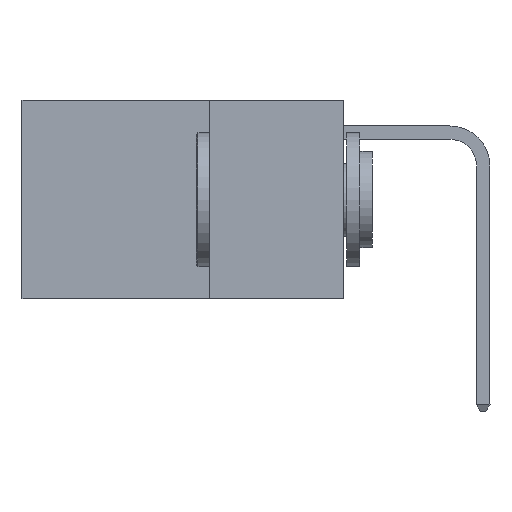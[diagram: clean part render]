
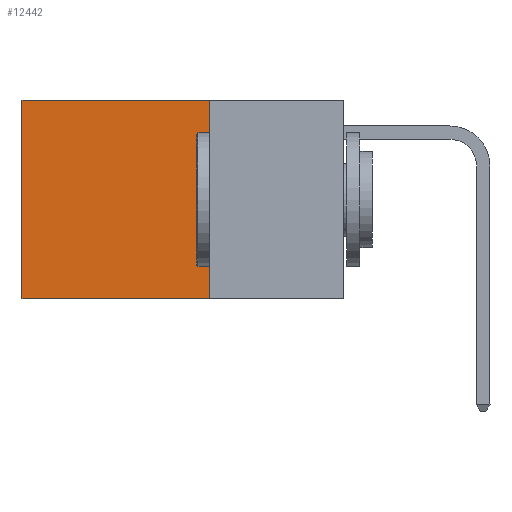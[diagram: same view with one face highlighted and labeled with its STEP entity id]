
A CAD part, left-side view. The second image highlights one B-rep face of the part: STEP entity #12442.
In plain terms, the highlighted planar face has unit normal (-1, 0, 0).
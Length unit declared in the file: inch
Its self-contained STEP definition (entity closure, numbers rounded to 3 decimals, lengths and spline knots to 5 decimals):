
#922 = EDGE_CURVE ( 'NONE', #7357, #18451, #21906, .T. ) ;
#1188 = DIRECTION ( 'NONE',  ( 0., 1., 0. ) ) ;
#1688 = EDGE_CURVE ( 'NONE', #15909, #7357, #16612, .T. ) ;
#2208 = EDGE_CURVE ( 'NONE', #21267, #18451, #7711, .T. ) ;
#3041 = DIRECTION ( 'NONE',  ( 1., 0., 0. ) ) ;
#3292 = VECTOR ( 'NONE', #18021, 39.37008 ) ;
#3770 = CARTESIAN_POINT ( 'NONE',  ( 0.2625, 0.25, -0.37 ) ) ;
#4012 = CARTESIAN_POINT ( 'NONE',  ( 0.2625, 0.6, 0. ) ) ;
#4087 = VECTOR ( 'NONE', #1188, 39.37008 ) ;
#7357 = VERTEX_POINT ( 'NONE', #25743 ) ;
#7711 = LINE ( 'NONE', #3770, #11055 ) ;
#10145 = AXIS2_PLACEMENT_3D ( 'NONE', #15084, #3041, #21061 ) ;
#10602 = ORIENTED_EDGE ( 'NONE', *, *, #922, .T. ) ;
#11055 = VECTOR ( 'NONE', #19711, 39.37008 ) ;
#12121 = EDGE_LOOP ( 'NONE', ( #10602, #19441, #14512, #16993 ) ) ;
#12442 = ADVANCED_FACE ( 'NONE', ( #20928 ), #23022, .F. ) ;
#14097 = DIRECTION ( 'NONE',  ( 0., 0., -1. ) ) ;
#14512 = ORIENTED_EDGE ( 'NONE', *, *, #14636, .F. ) ;
#14636 = EDGE_CURVE ( 'NONE', #15909, #21267, #24122, .T. ) ;
#15084 = CARTESIAN_POINT ( 'NONE',  ( 0.2625, 0.25, 0. ) ) ;
#15909 = VERTEX_POINT ( 'NONE', #19842 ) ;
#16612 = LINE ( 'NONE', #18699, #4087 ) ;
#16993 = ORIENTED_EDGE ( 'NONE', *, *, #1688, .T. ) ;
#18021 = DIRECTION ( 'NONE',  ( 0., 0., -1. ) ) ;
#18087 = VECTOR ( 'NONE', #14097, 39.37008 ) ;
#18399 = CARTESIAN_POINT ( 'NONE',  ( 0.2625, 0.25, 0. ) ) ;
#18451 = VERTEX_POINT ( 'NONE', #23750 ) ;
#18699 = CARTESIAN_POINT ( 'NONE',  ( 0.2625, 0.25, 0. ) ) ;
#19441 = ORIENTED_EDGE ( 'NONE', *, *, #2208, .F. ) ;
#19711 = DIRECTION ( 'NONE',  ( 0., 1., 0. ) ) ;
#19842 = CARTESIAN_POINT ( 'NONE',  ( 0.2625, 0.25, 0. ) ) ;
#20928 = FACE_OUTER_BOUND ( 'NONE', #12121, .T. ) ;
#21061 = DIRECTION ( 'NONE',  ( 0., 0., -1. ) ) ;
#21267 = VERTEX_POINT ( 'NONE', #25737 ) ;
#21906 = LINE ( 'NONE', #4012, #3292 ) ;
#23022 = PLANE ( 'NONE',  #10145 ) ;
#23750 = CARTESIAN_POINT ( 'NONE',  ( 0.2625, 0.6, -0.37 ) ) ;
#24122 = LINE ( 'NONE', #18399, #18087 ) ;
#25737 = CARTESIAN_POINT ( 'NONE',  ( 0.2625, 0.25, -0.37 ) ) ;
#25743 = CARTESIAN_POINT ( 'NONE',  ( 0.2625, 0.6, 0. ) ) ;
